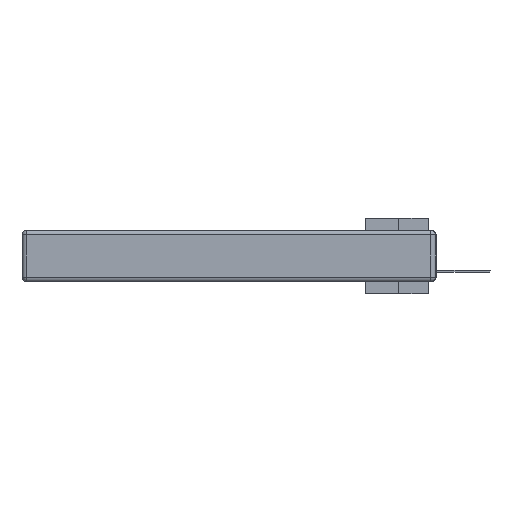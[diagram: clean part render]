
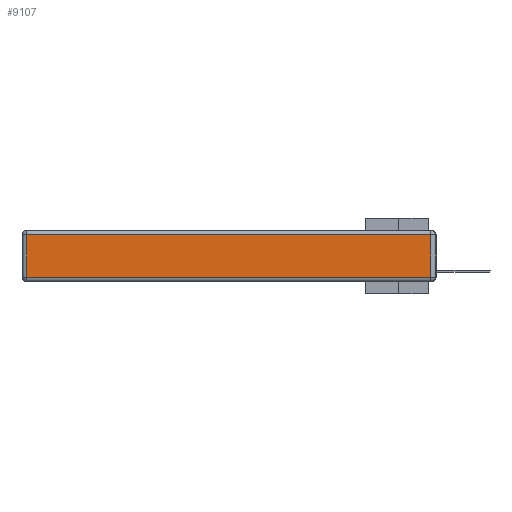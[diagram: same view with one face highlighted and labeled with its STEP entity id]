
A CAD part, left-side view. The second image highlights one B-rep face of the part: STEP entity #9107.
In plain terms, the highlighted planar face has unit normal (-1, 0, 0).
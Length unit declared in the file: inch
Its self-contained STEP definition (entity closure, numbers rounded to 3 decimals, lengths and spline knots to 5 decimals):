
#1505 = CARTESIAN_POINT ( 'NONE',  ( 0., 2.75, -0.03 ) ) ;
#2411 = VECTOR ( 'NONE', #18149, 39.37008 ) ;
#3428 = VERTEX_POINT ( 'NONE', #24768 ) ;
#3455 = VERTEX_POINT ( 'NONE', #27161 ) ;
#3583 = DIRECTION ( 'NONE',  ( 0., 0., 1. ) ) ;
#4505 = VECTOR ( 'NONE', #10276, 39.37008 ) ;
#5782 = EDGE_CURVE ( 'NONE', #18462, #3428, #22707, .T. ) ;
#6040 = ORIENTED_EDGE ( 'NONE', *, *, #10519, .T. ) ;
#6605 = ORIENTED_EDGE ( 'NONE', *, *, #20611, .T. ) ;
#6711 = CARTESIAN_POINT ( 'NONE',  ( 0., 0., -0.313 ) ) ;
#6915 = DIRECTION ( 'NONE',  ( 0., -1., 0. ) ) ;
#7395 = AXIS2_PLACEMENT_3D ( 'NONE', #7925, #27654, #3583 ) ;
#7826 = PLANE ( 'NONE',  #7395 ) ;
#7925 = CARTESIAN_POINT ( 'NONE',  ( 0., 0., -0.343 ) ) ;
#8295 = CARTESIAN_POINT ( 'NONE',  ( 0., 0.03, -0.03 ) ) ;
#9107 = ADVANCED_FACE ( 'NONE', ( #15030 ), #7826, .T. ) ;
#10246 = CARTESIAN_POINT ( 'NONE',  ( 0., 0.03, -0.313 ) ) ;
#10276 = DIRECTION ( 'NONE',  ( 0., 1., 0. ) ) ;
#10519 = EDGE_CURVE ( 'NONE', #3428, #3455, #11115, .T. ) ;
#11115 = LINE ( 'NONE', #17253, #22093 ) ;
#15030 = FACE_OUTER_BOUND ( 'NONE', #18953, .T. ) ;
#15671 = EDGE_CURVE ( 'NONE', #3455, #20755, #23349, .T. ) ;
#17253 = CARTESIAN_POINT ( 'NONE',  ( 0., 2.72, -0.343 ) ) ;
#18149 = DIRECTION ( 'NONE',  ( 0., 0., 1. ) ) ;
#18462 = VERTEX_POINT ( 'NONE', #8295 ) ;
#18953 = EDGE_LOOP ( 'NONE', ( #20666, #6605, #20295, #6040 ) ) ;
#20295 = ORIENTED_EDGE ( 'NONE', *, *, #5782, .T. ) ;
#20611 = EDGE_CURVE ( 'NONE', #20755, #18462, #26759, .T. ) ;
#20666 = ORIENTED_EDGE ( 'NONE', *, *, #15671, .T. ) ;
#20755 = VERTEX_POINT ( 'NONE', #10246 ) ;
#22093 = VECTOR ( 'NONE', #23943, 39.37008 ) ;
#22707 = LINE ( 'NONE', #1505, #4505 ) ;
#23349 = LINE ( 'NONE', #6711, #23712 ) ;
#23712 = VECTOR ( 'NONE', #6915, 39.37008 ) ;
#23943 = DIRECTION ( 'NONE',  ( 0., 0., -1. ) ) ;
#24768 = CARTESIAN_POINT ( 'NONE',  ( 0., 2.72, -0.03 ) ) ;
#26759 = LINE ( 'NONE', #26775, #2411 ) ;
#26775 = CARTESIAN_POINT ( 'NONE',  ( 0., 0.03, -0.343 ) ) ;
#27161 = CARTESIAN_POINT ( 'NONE',  ( 0., 2.72, -0.313 ) ) ;
#27654 = DIRECTION ( 'NONE',  ( -1., 0., 0. ) ) ;
